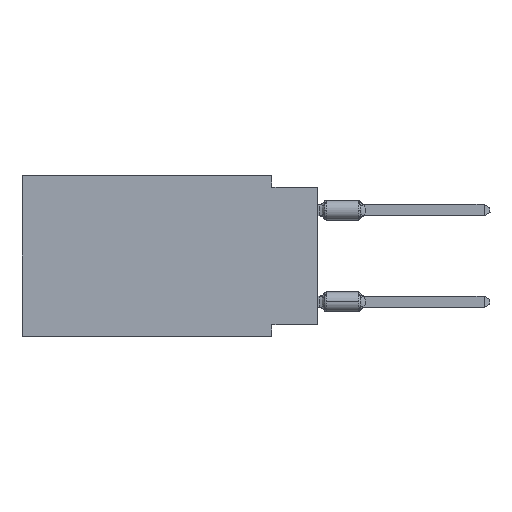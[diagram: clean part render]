
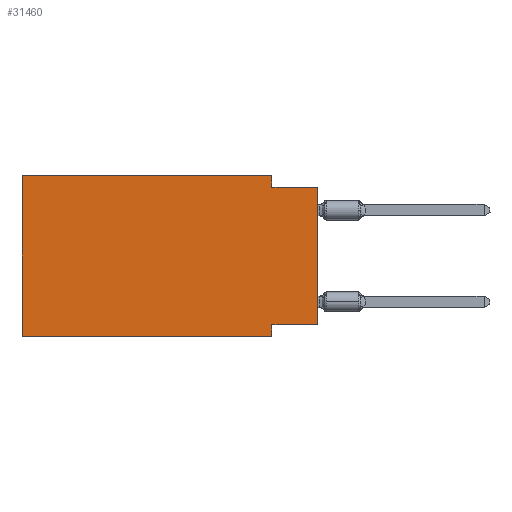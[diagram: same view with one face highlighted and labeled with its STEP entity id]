
A CAD part, left-side view. The second image highlights one B-rep face of the part: STEP entity #31460.
In plain terms, the highlighted planar face has unit normal (-1, 0, 0).
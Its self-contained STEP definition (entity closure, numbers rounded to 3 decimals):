
#1206 = DIRECTION ( 'NONE',  ( 0., -1., 0. ) ) ;
#3033 = ORIENTED_EDGE ( 'NONE', *, *, #20587, .F. ) ;
#4055 = ORIENTED_EDGE ( 'NONE', *, *, #60647, .F. ) ;
#6834 = DIRECTION ( 'NONE',  ( 1., 0., 0. ) ) ;
#7323 = EDGE_CURVE ( 'NONE', #60716, #9889, #27295, .T. ) ;
#7770 = DIRECTION ( 'NONE',  ( 0., 1., 0. ) ) ;
#8680 = EDGE_CURVE ( 'NONE', #9889, #59775, #28701, .T. ) ;
#9834 = VECTOR ( 'NONE', #7770, 1000. ) ;
#9889 = VERTEX_POINT ( 'NONE', #29961 ) ;
#11431 = DIRECTION ( 'NONE',  ( 0., 0., -1. ) ) ;
#12278 = VERTEX_POINT ( 'NONE', #24241 ) ;
#12521 = VECTOR ( 'NONE', #1206, 1000. ) ;
#15897 = LINE ( 'NONE', #21613, #27365 ) ;
#16698 = VECTOR ( 'NONE', #42707, 1000. ) ;
#17325 = LINE ( 'NONE', #36744, #9834 ) ;
#19048 = CARTESIAN_POINT ( 'NONE',  ( 0., 2.54, -8.89 ) ) ;
#19145 = CARTESIAN_POINT ( 'NONE',  ( 0., 2.54, 0. ) ) ;
#19566 = CARTESIAN_POINT ( 'NONE',  ( 0., 2.54, -0.635 ) ) ;
#20441 = LINE ( 'NONE', #54851, #22885 ) ;
#20587 = EDGE_CURVE ( 'NONE', #48677, #62100, #17325, .T. ) ;
#21613 = CARTESIAN_POINT ( 'NONE',  ( 0., 2.54, -8.89 ) ) ;
#21800 = FACE_OUTER_BOUND ( 'NONE', #32618, .T. ) ;
#22885 = VECTOR ( 'NONE', #40508, 1000. ) ;
#24241 = CARTESIAN_POINT ( 'NONE',  ( 0., 0., -0.635 ) ) ;
#25248 = VECTOR ( 'NONE', #43390, 1000. ) ;
#26799 = EDGE_CURVE ( 'NONE', #59775, #12278, #54087, .T. ) ;
#27295 = LINE ( 'NONE', #61393, #50807 ) ;
#27365 = VECTOR ( 'NONE', #11431, 1000. ) ;
#27588 = EDGE_CURVE ( 'NONE', #34193, #60716, #56421, .T. ) ;
#28701 = LINE ( 'NONE', #19145, #59041 ) ;
#29008 = EDGE_CURVE ( 'NONE', #48677, #12278, #20441, .T. ) ;
#29875 = CARTESIAN_POINT ( 'NONE',  ( 0., 0., -0.635 ) ) ;
#29961 = CARTESIAN_POINT ( 'NONE',  ( 0., 2.54, 0. ) ) ;
#29973 = LINE ( 'NONE', #38912, #25248 ) ;
#31460 = ADVANCED_FACE ( 'NONE', ( #21800 ), #46968, .F. ) ;
#32470 = VERTEX_POINT ( 'NONE', #19048 ) ;
#32618 = EDGE_LOOP ( 'NONE', ( #35243, #52577, #54345, #49014, #48922, #37330, #4055, #3033 ) ) ;
#34193 = VERTEX_POINT ( 'NONE', #43511 ) ;
#35158 = AXIS2_PLACEMENT_3D ( 'NONE', #46019, #6834, #51737 ) ;
#35243 = ORIENTED_EDGE ( 'NONE', *, *, #29008, .T. ) ;
#35634 = CARTESIAN_POINT ( 'NONE',  ( 0., 16.383, 0. ) ) ;
#36744 = CARTESIAN_POINT ( 'NONE',  ( 0., 0., -8.255 ) ) ;
#37158 = DIRECTION ( 'NONE',  ( 0., -1., 0. ) ) ;
#37330 = ORIENTED_EDGE ( 'NONE', *, *, #49067, .T. ) ;
#38912 = CARTESIAN_POINT ( 'NONE',  ( 0., 16.383, -8.89 ) ) ;
#40508 = DIRECTION ( 'NONE',  ( 0., 0., 1. ) ) ;
#42707 = DIRECTION ( 'NONE',  ( 0., 0., 1. ) ) ;
#43343 = CARTESIAN_POINT ( 'NONE',  ( 0., 16.383, 0. ) ) ;
#43390 = DIRECTION ( 'NONE',  ( 0., -1., 0. ) ) ;
#43511 = CARTESIAN_POINT ( 'NONE',  ( 0., 16.383, -8.89 ) ) ;
#43879 = CARTESIAN_POINT ( 'NONE',  ( 0., 2.54, -8.255 ) ) ;
#46019 = CARTESIAN_POINT ( 'NONE',  ( 0., 16.383, 0. ) ) ;
#46968 = PLANE ( 'NONE',  #35158 ) ;
#48459 = DIRECTION ( 'NONE',  ( 0., 0., -1. ) ) ;
#48677 = VERTEX_POINT ( 'NONE', #49485 ) ;
#48922 = ORIENTED_EDGE ( 'NONE', *, *, #27588, .F. ) ;
#49014 = ORIENTED_EDGE ( 'NONE', *, *, #7323, .F. ) ;
#49067 = EDGE_CURVE ( 'NONE', #34193, #32470, #29973, .T. ) ;
#49485 = CARTESIAN_POINT ( 'NONE',  ( 0., 0., -8.255 ) ) ;
#50807 = VECTOR ( 'NONE', #37158, 1000. ) ;
#51737 = DIRECTION ( 'NONE',  ( 0., 0., -1. ) ) ;
#52577 = ORIENTED_EDGE ( 'NONE', *, *, #26799, .F. ) ;
#54087 = LINE ( 'NONE', #29875, #12521 ) ;
#54345 = ORIENTED_EDGE ( 'NONE', *, *, #8680, .F. ) ;
#54851 = CARTESIAN_POINT ( 'NONE',  ( 0., 0., 0. ) ) ;
#56421 = LINE ( 'NONE', #43343, #16698 ) ;
#59041 = VECTOR ( 'NONE', #48459, 1000. ) ;
#59775 = VERTEX_POINT ( 'NONE', #19566 ) ;
#60647 = EDGE_CURVE ( 'NONE', #62100, #32470, #15897, .T. ) ;
#60716 = VERTEX_POINT ( 'NONE', #35634 ) ;
#61393 = CARTESIAN_POINT ( 'NONE',  ( 0., 16.383, 0. ) ) ;
#62100 = VERTEX_POINT ( 'NONE', #43879 ) ;
